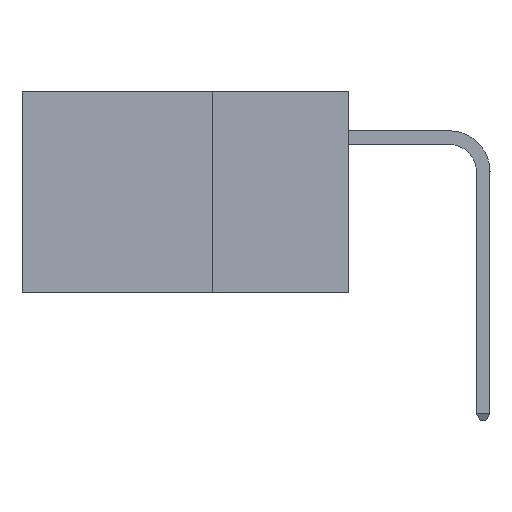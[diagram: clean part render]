
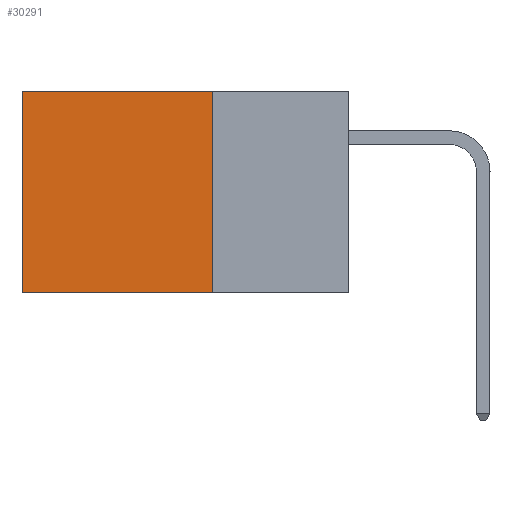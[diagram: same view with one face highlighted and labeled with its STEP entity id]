
A CAD part, left-side view. The second image highlights one B-rep face of the part: STEP entity #30291.
In plain terms, the highlighted planar face has unit normal (-1, 0, 0).
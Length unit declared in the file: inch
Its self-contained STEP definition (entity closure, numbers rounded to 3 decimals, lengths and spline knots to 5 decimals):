
#595 = EDGE_CURVE ( 'NONE', #9343, #25468, #29008, .T. ) ;
#883 = ORIENTED_EDGE ( 'NONE', *, *, #595, .T. ) ;
#2969 = LINE ( 'NONE', #8960, #27891 ) ;
#3478 = VERTEX_POINT ( 'NONE', #7369 ) ;
#3734 = VERTEX_POINT ( 'NONE', #20977 ) ;
#4563 = ORIENTED_EDGE ( 'NONE', *, *, #37186, .F. ) ;
#5977 = ORIENTED_EDGE ( 'NONE', *, *, #25821, .T. ) ;
#7369 = CARTESIAN_POINT ( 'NONE',  ( 0.2875, 0.6, -0.37 ) ) ;
#8270 = LINE ( 'NONE', #32013, #33070 ) ;
#8819 = EDGE_CURVE ( 'NONE', #9343, #3734, #26618, .T. ) ;
#8960 = CARTESIAN_POINT ( 'NONE',  ( 0.2875, 0.6, 0. ) ) ;
#9343 = VERTEX_POINT ( 'NONE', #25167 ) ;
#11986 = DIRECTION ( 'NONE',  ( 0., 1., 0. ) ) ;
#13788 = CARTESIAN_POINT ( 'NONE',  ( 0.2875, 0.25, 0. ) ) ;
#13919 = CARTESIAN_POINT ( 'NONE',  ( 0.2875, 0.25, 0. ) ) ;
#13921 = DIRECTION ( 'NONE',  ( 1., 0., 0. ) ) ;
#16188 = CARTESIAN_POINT ( 'NONE',  ( 0.2875, 0.25, 0. ) ) ;
#16533 = DIRECTION ( 'NONE',  ( 0., 1., 0. ) ) ;
#19322 = DIRECTION ( 'NONE',  ( 0., 0., -1. ) ) ;
#20699 = VECTOR ( 'NONE', #11986, 39.37008 ) ;
#20977 = CARTESIAN_POINT ( 'NONE',  ( 0.2875, 0.25, -0.37 ) ) ;
#25167 = CARTESIAN_POINT ( 'NONE',  ( 0.2875, 0.25, 0. ) ) ;
#25468 = VERTEX_POINT ( 'NONE', #25884 ) ;
#25821 = EDGE_CURVE ( 'NONE', #25468, #3478, #2969, .T. ) ;
#25884 = CARTESIAN_POINT ( 'NONE',  ( 0.2875, 0.6, 0. ) ) ;
#26618 = LINE ( 'NONE', #16188, #35818 ) ;
#27891 = VECTOR ( 'NONE', #30697, 39.37008 ) ;
#29008 = LINE ( 'NONE', #13919, #20699 ) ;
#30291 = ADVANCED_FACE ( 'NONE', ( #35453 ), #38642, .F. ) ;
#30697 = DIRECTION ( 'NONE',  ( 0., 0., -1. ) ) ;
#32013 = CARTESIAN_POINT ( 'NONE',  ( 0.2875, 0.25, -0.37 ) ) ;
#32151 = AXIS2_PLACEMENT_3D ( 'NONE', #13788, #13921, #35667 ) ;
#33070 = VECTOR ( 'NONE', #16533, 39.37008 ) ;
#33658 = EDGE_LOOP ( 'NONE', ( #5977, #4563, #35218, #883 ) ) ;
#35218 = ORIENTED_EDGE ( 'NONE', *, *, #8819, .F. ) ;
#35453 = FACE_OUTER_BOUND ( 'NONE', #33658, .T. ) ;
#35667 = DIRECTION ( 'NONE',  ( 0., 0., -1. ) ) ;
#35818 = VECTOR ( 'NONE', #19322, 39.37008 ) ;
#37186 = EDGE_CURVE ( 'NONE', #3734, #3478, #8270, .T. ) ;
#38642 = PLANE ( 'NONE',  #32151 ) ;
